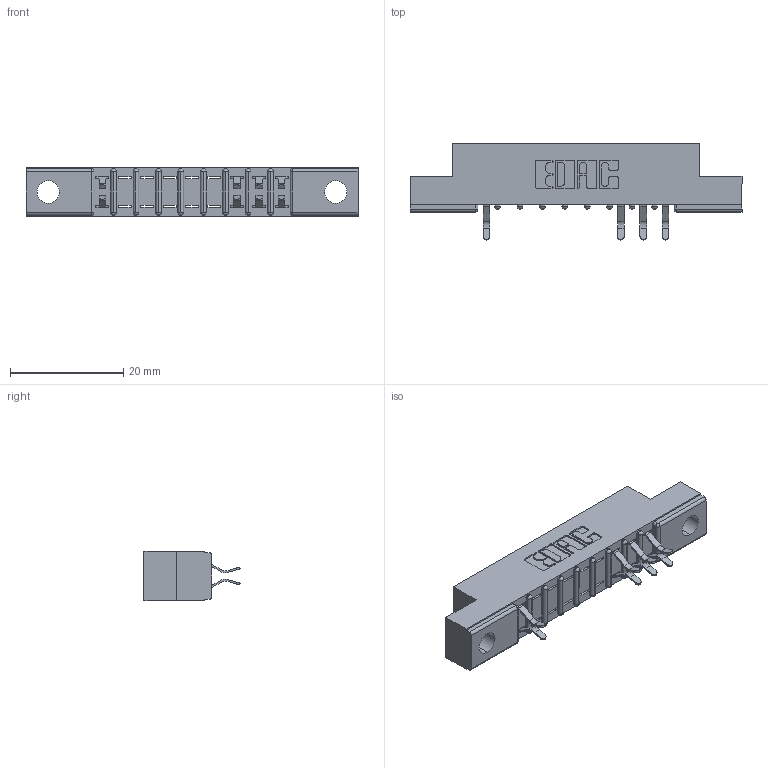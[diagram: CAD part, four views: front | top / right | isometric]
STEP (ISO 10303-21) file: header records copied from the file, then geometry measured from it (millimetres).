
FILE_DESCRIPTION (( 'STEP AP203' ), '1' );
FILE_NAME ('357-018-556-204.STEP', '2018-08-08T05:47:02', ( '' ), ( '' ), 'SwSTEP 2.0', 'SolidWorks 2016', '' );
FILE_SCHEMA (( 'CONFIG_CONTROL_DESIGN' ));
Length unit declared in the file: inch
Products named in the file (3): 307-290-001_556; 357-018-556-204; 307 Part_.156 Dia Mounting Holes
Assembly tree (9 placements, depth 2):
  357-018-556-204
    307 Part_.156 Dia Mounting Holes
    307-290-001_556  x8
Bounding box: 58.67 x 16.97 x 8.71 mm (x, y, z)
Volume: 3602.5 mm3; surface area: 4800.8 mm2
Topology: 9 solids, 9 shells, 642 faces, 1815 edges, 1170 vertices
Faces by surface type: plane 408, cylinder 214, sphere 20
Entity records: 12274 total; most frequent: CARTESIAN_POINT 2065, ORIENTED_EDGE 2050, DIRECTION 2019, EDGE_CURVE 1025, LINE 779, VECTOR 779, VERTEX_POINT 666, AXIS2_PLACEMENT_3D 620
